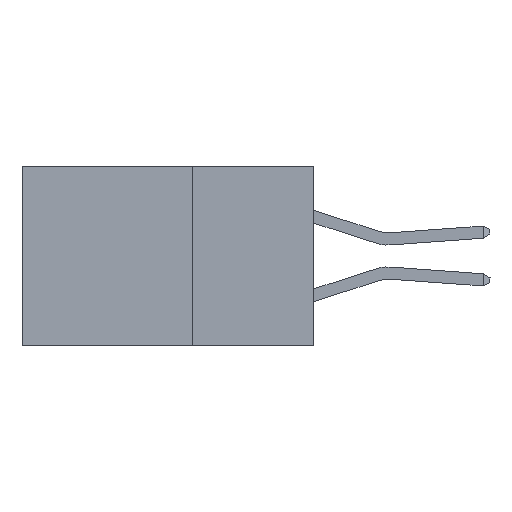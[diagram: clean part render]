
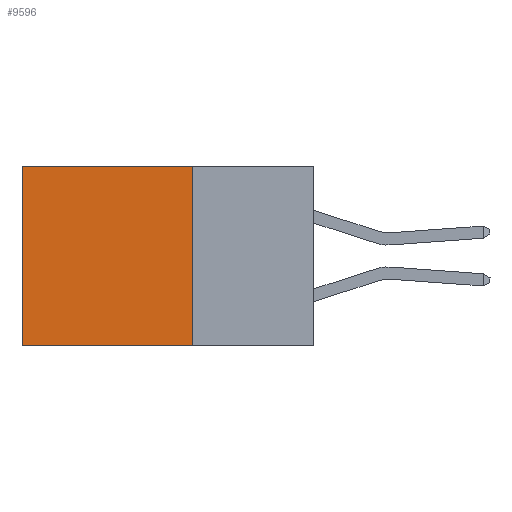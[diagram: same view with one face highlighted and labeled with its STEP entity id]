
A CAD part, left-side view. The second image highlights one B-rep face of the part: STEP entity #9596.
In plain terms, the highlighted planar face has unit normal (-1, 0, 0).
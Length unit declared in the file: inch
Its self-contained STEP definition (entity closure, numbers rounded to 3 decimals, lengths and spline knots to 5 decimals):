
#38 = EDGE_CURVE ( 'NONE', #9145, #5735, #1506, .T. ) ;
#453 = CARTESIAN_POINT ( 'NONE',  ( 0.2875, 0.25, -0.37 ) ) ;
#879 = CARTESIAN_POINT ( 'NONE',  ( 0.2875, 0.6, 0. ) ) ;
#1009 = ORIENTED_EDGE ( 'NONE', *, *, #4994, .T. ) ;
#1201 = LINE ( 'NONE', #2602, #1332 ) ;
#1285 = EDGE_LOOP ( 'NONE', ( #7105, #6837, #2871, #1009 ) ) ;
#1332 = VECTOR ( 'NONE', #9750, 39.37008 ) ;
#1506 = LINE ( 'NONE', #8680, #6829 ) ;
#1689 = VECTOR ( 'NONE', #2460, 39.37008 ) ;
#2070 = DIRECTION ( 'NONE',  ( 0., 1., 0. ) ) ;
#2144 = VERTEX_POINT ( 'NONE', #9007 ) ;
#2288 = CARTESIAN_POINT ( 'NONE',  ( 0.2875, 0.6, -0.37 ) ) ;
#2460 = DIRECTION ( 'NONE',  ( 0., 1., 0. ) ) ;
#2602 = CARTESIAN_POINT ( 'NONE',  ( 0.2875, 0.25, 0. ) ) ;
#2871 = ORIENTED_EDGE ( 'NONE', *, *, #4099, .F. ) ;
#2915 = DIRECTION ( 'NONE',  ( 0., 0., -1. ) ) ;
#3079 = LINE ( 'NONE', #7048, #1689 ) ;
#3859 = CARTESIAN_POINT ( 'NONE',  ( 0.2875, 0.25, 0. ) ) ;
#3955 = DIRECTION ( 'NONE',  ( 0., 0., -1. ) ) ;
#4099 = EDGE_CURVE ( 'NONE', #2144, #6137, #1201, .T. ) ;
#4394 = CARTESIAN_POINT ( 'NONE',  ( 0.2875, 0.25, -0.37 ) ) ;
#4994 = EDGE_CURVE ( 'NONE', #2144, #9145, #3079, .T. ) ;
#5228 = PLANE ( 'NONE',  #6311 ) ;
#5274 = VECTOR ( 'NONE', #2070, 39.37008 ) ;
#5735 = VERTEX_POINT ( 'NONE', #2288 ) ;
#6062 = DIRECTION ( 'NONE',  ( 1., 0., 0. ) ) ;
#6137 = VERTEX_POINT ( 'NONE', #4394 ) ;
#6311 = AXIS2_PLACEMENT_3D ( 'NONE', #3859, #6062, #2915 ) ;
#6829 = VECTOR ( 'NONE', #3955, 39.37008 ) ;
#6837 = ORIENTED_EDGE ( 'NONE', *, *, #8623, .F. ) ;
#7048 = CARTESIAN_POINT ( 'NONE',  ( 0.2875, 0.25, 0. ) ) ;
#7105 = ORIENTED_EDGE ( 'NONE', *, *, #38, .T. ) ;
#8433 = FACE_OUTER_BOUND ( 'NONE', #1285, .T. ) ;
#8623 = EDGE_CURVE ( 'NONE', #6137, #5735, #8847, .T. ) ;
#8680 = CARTESIAN_POINT ( 'NONE',  ( 0.2875, 0.6, 0. ) ) ;
#8847 = LINE ( 'NONE', #453, #5274 ) ;
#9007 = CARTESIAN_POINT ( 'NONE',  ( 0.2875, 0.25, 0. ) ) ;
#9145 = VERTEX_POINT ( 'NONE', #879 ) ;
#9596 = ADVANCED_FACE ( 'NONE', ( #8433 ), #5228, .F. ) ;
#9750 = DIRECTION ( 'NONE',  ( 0., 0., -1. ) ) ;
